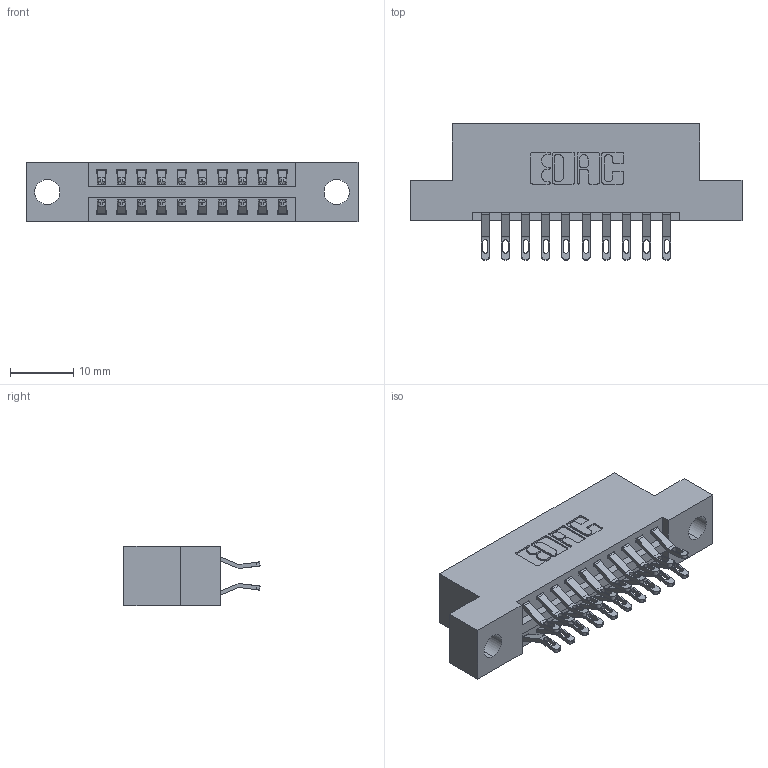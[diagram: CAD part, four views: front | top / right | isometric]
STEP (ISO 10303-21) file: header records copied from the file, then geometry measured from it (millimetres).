
FILE_DESCRIPTION (( 'STEP AP203' ), '1' );
FILE_NAME ('346-020-555-204.STEP', '2022-05-18T19:36:22', ( '' ), ( '' ), 'SwSTEP 2.0', 'SolidWorks 2020', '' );
FILE_SCHEMA (( 'CONFIG_CONTROL_DESIGN' ));
Length unit declared in the file: inch
Products named in the file (3): 346 Part_Flush Mounting Lugs - 0.156 Dia-TH; 346-020-555-204; 345-292-001_555 Tail
Assembly tree (21 placements, depth 2):
  346-020-555-204
    346 Part_Flush Mounting Lugs - 0.156 Dia-TH
    345-292-001_555 Tail  x20
Bounding box: 52.32 x 21.46 x 9.4 mm (x, y, z)
Volume: 4805.8 mm3; surface area: 6157.6 mm2
Topology: 21 solids, 21 shells, 1296 faces, 4025 edges, 2682 vertices
Faces by surface type: plane 750, cylinder 546
Entity records: 11579 total; most frequent: CARTESIAN_POINT 1992, ORIENTED_EDGE 1894, DIRECTION 1775, EDGE_CURVE 947, VECTOR 755, LINE 755, VERTEX_POINT 630, AXIS2_PLACEMENT_3D 510
